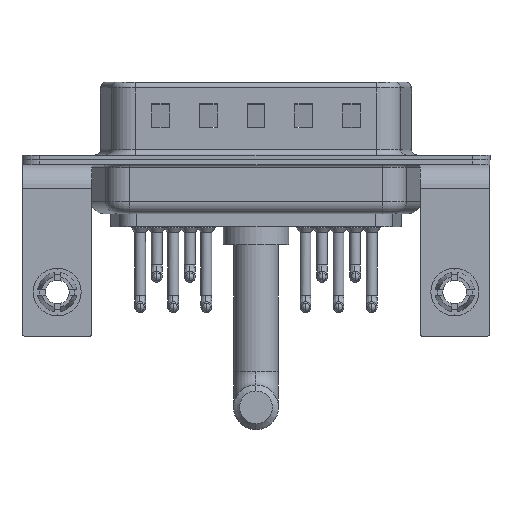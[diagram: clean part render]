
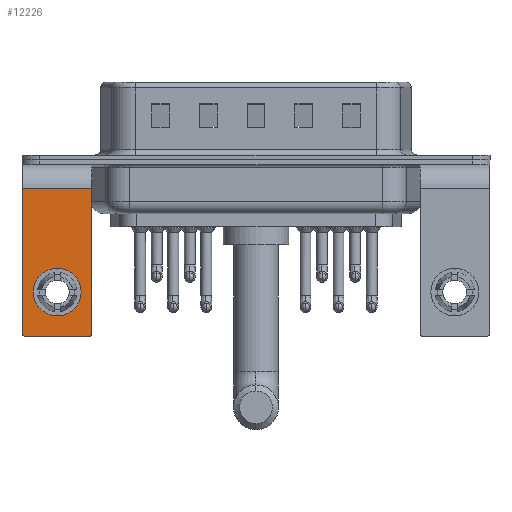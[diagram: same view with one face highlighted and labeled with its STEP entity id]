
A CAD part, front view. The second image highlights one B-rep face of the part: STEP entity #12226.
In plain terms, the highlighted planar face has unit normal (0, -1, 0).
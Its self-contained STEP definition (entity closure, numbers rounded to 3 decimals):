
#152 = FACE_OUTER_BOUND ( 'NONE', #1122, .T. ) ;
#246 = CIRCLE ( 'NONE', #18402, 2. ) ;
#602 = VECTOR ( 'NONE', #3570, 1000. ) ;
#741 = LINE ( 'NONE', #16139, #13134 ) ;
#1122 = EDGE_LOOP ( 'NONE', ( #23304, #22014, #4731, #17710, #5727, #3237 ) ) ;
#1545 = LINE ( 'NONE', #15052, #602 ) ;
#1828 = VERTEX_POINT ( 'NONE', #23864 ) ;
#1947 = ORIENTED_EDGE ( 'NONE', *, *, #6768, .T. ) ;
#2064 = FACE_BOUND ( 'NONE', #11525, .T. ) ;
#2399 = DIRECTION ( 'NONE',  ( 0., 1., 0. ) ) ;
#2526 = EDGE_CURVE ( 'NONE', #9784, #8326, #13590, .T. ) ;
#3237 = ORIENTED_EDGE ( 'NONE', *, *, #19333, .T. ) ;
#3570 = DIRECTION ( 'NONE',  ( -1., 0., 0. ) ) ;
#4105 = ORIENTED_EDGE ( 'NONE', *, *, #6844, .T. ) ;
#4731 = ORIENTED_EDGE ( 'NONE', *, *, #6700, .F. ) ;
#5449 = CARTESIAN_POINT ( 'NONE',  ( 2.65, -6.25, -14.55 ) ) ;
#5575 = DIRECTION ( 'NONE',  ( 0., -1., 0. ) ) ;
#5576 = DIRECTION ( 'NONE',  ( -1., 0., 0. ) ) ;
#5727 = ORIENTED_EDGE ( 'NONE', *, *, #23862, .F. ) ;
#5771 = DIRECTION ( 'NONE',  ( 0., 0., 1. ) ) ;
#6700 = EDGE_CURVE ( 'NONE', #8827, #8326, #24498, .T. ) ;
#6768 = EDGE_CURVE ( 'NONE', #8427, #22431, #246, .T. ) ;
#6844 = EDGE_CURVE ( 'NONE', #22431, #8427, #24044, .T. ) ;
#7233 = CARTESIAN_POINT ( 'NONE',  ( 2.9, -6.25, -14.8 ) ) ;
#7237 = AXIS2_PLACEMENT_3D ( 'NONE', #5449, #5575, #18683 ) ;
#7880 = DIRECTION ( 'NONE',  ( 0., 1., 0. ) ) ;
#8103 = DIRECTION ( 'NONE',  ( 0., 0., 1. ) ) ;
#8135 = CARTESIAN_POINT ( 'NONE',  ( 2.9, -6.25, -2.4 ) ) ;
#8326 = VERTEX_POINT ( 'NONE', #14022 ) ;
#8427 = VERTEX_POINT ( 'NONE', #12511 ) ;
#8827 = VERTEX_POINT ( 'NONE', #12354 ) ;
#9248 = CIRCLE ( 'NONE', #7237, 0.25 ) ;
#9459 = LINE ( 'NONE', #22949, #20912 ) ;
#9784 = VERTEX_POINT ( 'NONE', #21994 ) ;
#9894 = DIRECTION ( 'NONE',  ( 0., 0., 1. ) ) ;
#9905 = EDGE_CURVE ( 'NONE', #8827, #1828, #9248, .T. ) ;
#9965 = DIRECTION ( 'NONE',  ( 0., 0., -1. ) ) ;
#10346 = CARTESIAN_POINT ( 'NONE',  ( -2.9, -6.25, -2.4 ) ) ;
#11525 = EDGE_LOOP ( 'NONE', ( #1947, #4105 ) ) ;
#11627 = CARTESIAN_POINT ( 'NONE',  ( 0., -6.25, -11.07 ) ) ;
#11968 = VECTOR ( 'NONE', #5576, 1000. ) ;
#12002 = DIRECTION ( 'NONE',  ( 0., 1., 0. ) ) ;
#12226 = ADVANCED_FACE ( 'NONE', ( #2064, #152 ), #21373, .F. ) ;
#12354 = CARTESIAN_POINT ( 'NONE',  ( 2.65, -6.25, -14.8 ) ) ;
#12511 = CARTESIAN_POINT ( 'NONE',  ( 0., -6.25, -13.07 ) ) ;
#12883 = AXIS2_PLACEMENT_3D ( 'NONE', #8135, #7880, #9894 ) ;
#13134 = VECTOR ( 'NONE', #9965, 1000. ) ;
#13468 = DIRECTION ( 'NONE',  ( 0., -1., 0. ) ) ;
#13590 = CIRCLE ( 'NONE', #20844, 0.25 ) ;
#14022 = CARTESIAN_POINT ( 'NONE',  ( -2.65, -6.25, -14.8 ) ) ;
#14690 = VERTEX_POINT ( 'NONE', #10346 ) ;
#15052 = CARTESIAN_POINT ( 'NONE',  ( 2.9, -6.25, -2.4 ) ) ;
#15113 = CARTESIAN_POINT ( 'NONE',  ( -2.65, -6.25, -14.55 ) ) ;
#15381 = DIRECTION ( 'NONE',  ( 0., 0., -1. ) ) ;
#15900 = DIRECTION ( 'NONE',  ( 0., 0., 1. ) ) ;
#16139 = CARTESIAN_POINT ( 'NONE',  ( -2.9, -6.25, -2.4 ) ) ;
#17710 = ORIENTED_EDGE ( 'NONE', *, *, #9905, .T. ) ;
#18402 = AXIS2_PLACEMENT_3D ( 'NONE', #11627, #2399, #8103 ) ;
#18683 = DIRECTION ( 'NONE',  ( 0., 0., 1. ) ) ;
#18942 = CARTESIAN_POINT ( 'NONE',  ( 2.9, -6.25, -2.4 ) ) ;
#19215 = AXIS2_PLACEMENT_3D ( 'NONE', #19438, #12002, #15900 ) ;
#19333 = EDGE_CURVE ( 'NONE', #23268, #14690, #1545, .T. ) ;
#19438 = CARTESIAN_POINT ( 'NONE',  ( 0., -6.25, -11.07 ) ) ;
#19755 = CARTESIAN_POINT ( 'NONE',  ( 0., -6.25, -9.07 ) ) ;
#20134 = EDGE_CURVE ( 'NONE', #14690, #9784, #741, .T. ) ;
#20844 = AXIS2_PLACEMENT_3D ( 'NONE', #15113, #13468, #5771 ) ;
#20912 = VECTOR ( 'NONE', #15381, 1000. ) ;
#21373 = PLANE ( 'NONE',  #12883 ) ;
#21994 = CARTESIAN_POINT ( 'NONE',  ( -2.9, -6.25, -14.55 ) ) ;
#22014 = ORIENTED_EDGE ( 'NONE', *, *, #2526, .T. ) ;
#22431 = VERTEX_POINT ( 'NONE', #19755 ) ;
#22949 = CARTESIAN_POINT ( 'NONE',  ( 2.9, -6.25, -2.4 ) ) ;
#23268 = VERTEX_POINT ( 'NONE', #18942 ) ;
#23304 = ORIENTED_EDGE ( 'NONE', *, *, #20134, .T. ) ;
#23862 = EDGE_CURVE ( 'NONE', #23268, #1828, #9459, .T. ) ;
#23864 = CARTESIAN_POINT ( 'NONE',  ( 2.9, -6.25, -14.55 ) ) ;
#24044 = CIRCLE ( 'NONE', #19215, 2. ) ;
#24498 = LINE ( 'NONE', #7233, #11968 ) ;
